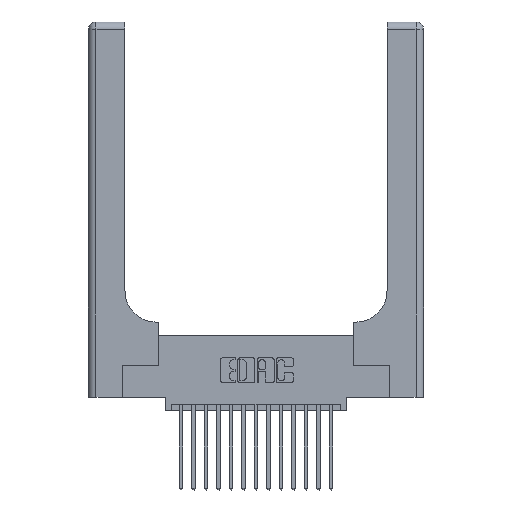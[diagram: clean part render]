
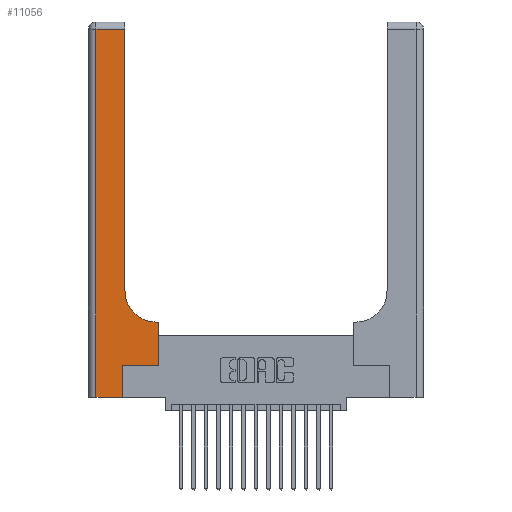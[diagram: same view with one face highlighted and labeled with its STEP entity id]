
A CAD part, top view. The second image highlights one B-rep face of the part: STEP entity #11056.
In plain terms, the highlighted planar face has unit normal (0, 0, 1).
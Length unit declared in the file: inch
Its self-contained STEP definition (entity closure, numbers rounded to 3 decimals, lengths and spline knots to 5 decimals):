
#49 = EDGE_LOOP ( 'NONE', ( #14546, #6189, #1373, #3542, #14614, #12223, #3657, #18487, #15256 ) ) ;
#415 = CARTESIAN_POINT ( 'NONE',  ( 0.2915, 2.94, 0.37 ) ) ;
#435 = DIRECTION ( 'NONE',  ( 1., 0., 0. ) ) ;
#1317 = VECTOR ( 'NONE', #17896, 39.37008 ) ;
#1373 = ORIENTED_EDGE ( 'NONE', *, *, #3973, .T. ) ;
#2573 = AXIS2_PLACEMENT_3D ( 'NONE', #3429, #13957, #4991 ) ;
#2786 = VECTOR ( 'NONE', #4165, 39.37008 ) ;
#2970 = EDGE_CURVE ( 'NONE', #11148, #12354, #10924, .T. ) ;
#3412 = AXIS2_PLACEMENT_3D ( 'NONE', #18425, #9741, #435 ) ;
#3429 = CARTESIAN_POINT ( 'NONE',  ( 0., 3., 0.37 ) ) ;
#3542 = ORIENTED_EDGE ( 'NONE', *, *, #9167, .T. ) ;
#3657 = ORIENTED_EDGE ( 'NONE', *, *, #13736, .T. ) ;
#3740 = LINE ( 'NONE', #12658, #19016 ) ;
#3741 = CARTESIAN_POINT ( 'NONE',  ( 0.5585, 0.25, 0.37 ) ) ;
#3958 = VECTOR ( 'NONE', #8526, 39.37008 ) ;
#3973 = EDGE_CURVE ( 'NONE', #12354, #7990, #3740, .T. ) ;
#4069 = LINE ( 'NONE', #13566, #1317 ) ;
#4110 = CARTESIAN_POINT ( 'NONE',  ( 0., 2.94, 0.37 ) ) ;
#4165 = DIRECTION ( 'NONE',  ( -1., 0., 0. ) ) ;
#4182 = LINE ( 'NONE', #4846, #16064 ) ;
#4354 = VERTEX_POINT ( 'NONE', #12378 ) ;
#4489 = EDGE_CURVE ( 'NONE', #18792, #8338, #7750, .T. ) ;
#4846 = CARTESIAN_POINT ( 'NONE',  ( 0.2915, 3., 0.37 ) ) ;
#4966 = EDGE_CURVE ( 'NONE', #8338, #11148, #4182, .T. ) ;
#4991 = DIRECTION ( 'NONE',  ( -1., 0., 0. ) ) ;
#5174 = EDGE_CURVE ( 'NONE', #17425, #15451, #12429, .T. ) ;
#5255 = CARTESIAN_POINT ( 'NONE',  ( 0.269, 0., 0.37 ) ) ;
#6055 = VECTOR ( 'NONE', #6317, 39.37008 ) ;
#6189 = ORIENTED_EDGE ( 'NONE', *, *, #2970, .T. ) ;
#6317 = DIRECTION ( 'NONE',  ( 1., 0., 0. ) ) ;
#6454 = PLANE ( 'NONE',  #2573 ) ;
#6483 = CARTESIAN_POINT ( 'NONE',  ( 0.06, 2.94, 0.37 ) ) ;
#7750 = CIRCLE ( 'NONE', #3412, 0.25 ) ;
#7990 = VERTEX_POINT ( 'NONE', #14833 ) ;
#8067 = LINE ( 'NONE', #16007, #11633 ) ;
#8192 = DIRECTION ( 'NONE',  ( 0., -1., 0. ) ) ;
#8338 = VERTEX_POINT ( 'NONE', #15637 ) ;
#8526 = DIRECTION ( 'NONE',  ( 1., 0., 0. ) ) ;
#9167 = EDGE_CURVE ( 'NONE', #7990, #17425, #15851, .T. ) ;
#9741 = DIRECTION ( 'NONE',  ( 0., 0., -1. ) ) ;
#10087 = CARTESIAN_POINT ( 'NONE',  ( 0.5415, 0.6, 0.37 ) ) ;
#10107 = LINE ( 'NONE', #10827, #6055 ) ;
#10827 = CARTESIAN_POINT ( 'NONE',  ( 0.269, 0.25, 0.37 ) ) ;
#10924 = LINE ( 'NONE', #4110, #2786 ) ;
#11056 = ADVANCED_FACE ( 'NONE', ( #12172 ), #6454, .F. ) ;
#11148 = VERTEX_POINT ( 'NONE', #415 ) ;
#11633 = VECTOR ( 'NONE', #17450, 39.37008 ) ;
#11757 = CARTESIAN_POINT ( 'NONE',  ( 0.269, 0.25, 0.37 ) ) ;
#12172 = FACE_OUTER_BOUND ( 'NONE', #49, .T. ) ;
#12223 = ORIENTED_EDGE ( 'NONE', *, *, #17898, .T. ) ;
#12354 = VERTEX_POINT ( 'NONE', #6483 ) ;
#12378 = CARTESIAN_POINT ( 'NONE',  ( 0.5585, 0.6, 0.37 ) ) ;
#12429 = LINE ( 'NONE', #5255, #15830 ) ;
#12658 = CARTESIAN_POINT ( 'NONE',  ( 0.06, 3., 0.37 ) ) ;
#13288 = EDGE_CURVE ( 'NONE', #4354, #18792, #4069, .T. ) ;
#13566 = CARTESIAN_POINT ( 'NONE',  ( 0.2915, 0.6, 0.37 ) ) ;
#13736 = EDGE_CURVE ( 'NONE', #17023, #4354, #8067, .T. ) ;
#13957 = DIRECTION ( 'NONE',  ( 0., 0., -1. ) ) ;
#14546 = ORIENTED_EDGE ( 'NONE', *, *, #4966, .T. ) ;
#14614 = ORIENTED_EDGE ( 'NONE', *, *, #5174, .T. ) ;
#14833 = CARTESIAN_POINT ( 'NONE',  ( 0.06, 0., 0.37 ) ) ;
#15256 = ORIENTED_EDGE ( 'NONE', *, *, #4489, .T. ) ;
#15264 = DIRECTION ( 'NONE',  ( 0., 1., 0. ) ) ;
#15451 = VERTEX_POINT ( 'NONE', #11757 ) ;
#15637 = CARTESIAN_POINT ( 'NONE',  ( 0.2915, 0.85, 0.37 ) ) ;
#15830 = VECTOR ( 'NONE', #18532, 39.37008 ) ;
#15851 = LINE ( 'NONE', #18751, #3958 ) ;
#16007 = CARTESIAN_POINT ( 'NONE',  ( 0.5585, 0.25, 0.37 ) ) ;
#16064 = VECTOR ( 'NONE', #15264, 39.37008 ) ;
#17023 = VERTEX_POINT ( 'NONE', #3741 ) ;
#17425 = VERTEX_POINT ( 'NONE', #18163 ) ;
#17450 = DIRECTION ( 'NONE',  ( 0., 1., 0. ) ) ;
#17896 = DIRECTION ( 'NONE',  ( -1., 0., 0. ) ) ;
#17898 = EDGE_CURVE ( 'NONE', #15451, #17023, #10107, .T. ) ;
#18163 = CARTESIAN_POINT ( 'NONE',  ( 0.269, 0., 0.37 ) ) ;
#18425 = CARTESIAN_POINT ( 'NONE',  ( 0.5415, 0.85, 0.37 ) ) ;
#18487 = ORIENTED_EDGE ( 'NONE', *, *, #13288, .T. ) ;
#18532 = DIRECTION ( 'NONE',  ( 0., 1., 0. ) ) ;
#18751 = CARTESIAN_POINT ( 'NONE',  ( 0., 0., 0.37 ) ) ;
#18792 = VERTEX_POINT ( 'NONE', #10087 ) ;
#19016 = VECTOR ( 'NONE', #8192, 39.37008 ) ;
